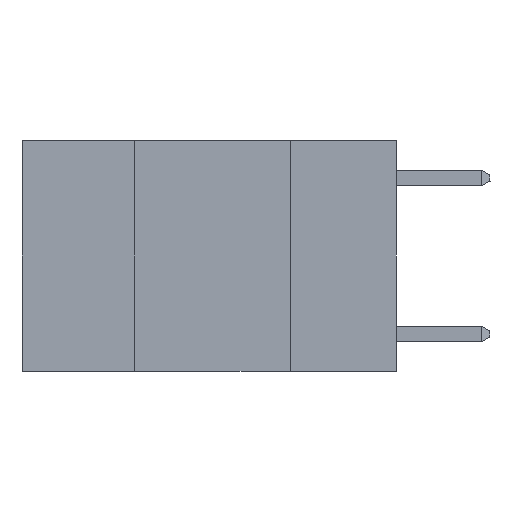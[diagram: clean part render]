
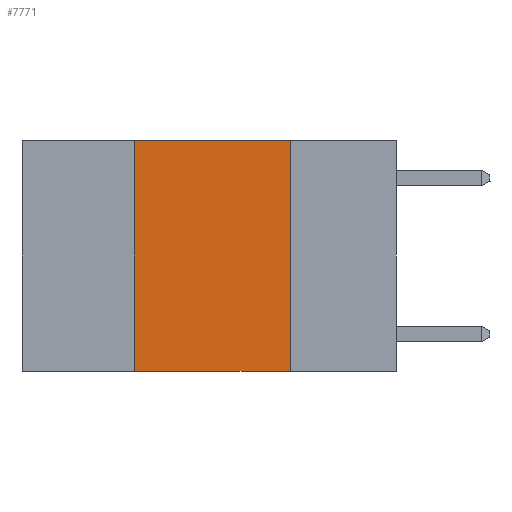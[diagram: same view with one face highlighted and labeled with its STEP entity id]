
A CAD part, left-side view. The second image highlights one B-rep face of the part: STEP entity #7771.
In plain terms, the highlighted planar face has unit normal (-1, 0, 0).
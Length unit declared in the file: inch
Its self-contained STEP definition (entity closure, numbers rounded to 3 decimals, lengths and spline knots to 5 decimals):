
#533 = VECTOR ( 'NONE', #6619, 39.37008 ) ;
#1297 = ORIENTED_EDGE ( 'NONE', *, *, #6411, .F. ) ;
#1954 = AXIS2_PLACEMENT_3D ( 'NONE', #7097, #7880, #3189 ) ;
#3022 = CARTESIAN_POINT ( 'NONE',  ( 0., 0.6, 0. ) ) ;
#3189 = DIRECTION ( 'NONE',  ( 0., 0., -1. ) ) ;
#3742 = CARTESIAN_POINT ( 'NONE',  ( 0., 0.17, 0. ) ) ;
#3816 = DIRECTION ( 'NONE',  ( 0., -1., 0. ) ) ;
#3895 = ORIENTED_EDGE ( 'NONE', *, *, #5168, .F. ) ;
#4308 = CARTESIAN_POINT ( 'NONE',  ( 0., 0.17, -0.37 ) ) ;
#4573 = CARTESIAN_POINT ( 'NONE',  ( 0., 0.42, -0.37 ) ) ;
#5168 = EDGE_CURVE ( 'NONE', #9447, #5591, #8827, .T. ) ;
#5373 = VECTOR ( 'NONE', #6586, 39.37008 ) ;
#5591 = VERTEX_POINT ( 'NONE', #7944 ) ;
#6292 = PLANE ( 'NONE',  #1954 ) ;
#6411 = EDGE_CURVE ( 'NONE', #6691, #8691, #9525, .T. ) ;
#6586 = DIRECTION ( 'NONE',  ( 0., 0., -1. ) ) ;
#6615 = LINE ( 'NONE', #8535, #8450 ) ;
#6619 = DIRECTION ( 'NONE',  ( 0., 0., 1. ) ) ;
#6690 = ORIENTED_EDGE ( 'NONE', *, *, #6727, .F. ) ;
#6691 = VERTEX_POINT ( 'NONE', #3742 ) ;
#6727 = EDGE_CURVE ( 'NONE', #5591, #6691, #7329, .T. ) ;
#7097 = CARTESIAN_POINT ( 'NONE',  ( 0., 0.6, 0. ) ) ;
#7329 = LINE ( 'NONE', #3022, #9159 ) ;
#7771 = ADVANCED_FACE ( 'NONE', ( #10121 ), #6292, .F. ) ;
#7880 = DIRECTION ( 'NONE',  ( 1., 0., 0. ) ) ;
#7944 = CARTESIAN_POINT ( 'NONE',  ( 0., 0.42, 0. ) ) ;
#8219 = EDGE_LOOP ( 'NONE', ( #1297, #6690, #3895, #9877 ) ) ;
#8450 = VECTOR ( 'NONE', #9308, 39.37008 ) ;
#8535 = CARTESIAN_POINT ( 'NONE',  ( 0., 0.6, -0.37 ) ) ;
#8691 = VERTEX_POINT ( 'NONE', #4308 ) ;
#8827 = LINE ( 'NONE', #8931, #533 ) ;
#8909 = CARTESIAN_POINT ( 'NONE',  ( 0., 0.17, 0. ) ) ;
#8931 = CARTESIAN_POINT ( 'NONE',  ( 0., 0.42, 0. ) ) ;
#9159 = VECTOR ( 'NONE', #3816, 39.37008 ) ;
#9308 = DIRECTION ( 'NONE',  ( 0., -1., 0. ) ) ;
#9447 = VERTEX_POINT ( 'NONE', #4573 ) ;
#9489 = EDGE_CURVE ( 'NONE', #9447, #8691, #6615, .T. ) ;
#9525 = LINE ( 'NONE', #8909, #5373 ) ;
#9877 = ORIENTED_EDGE ( 'NONE', *, *, #9489, .T. ) ;
#10121 = FACE_OUTER_BOUND ( 'NONE', #8219, .T. ) ;
